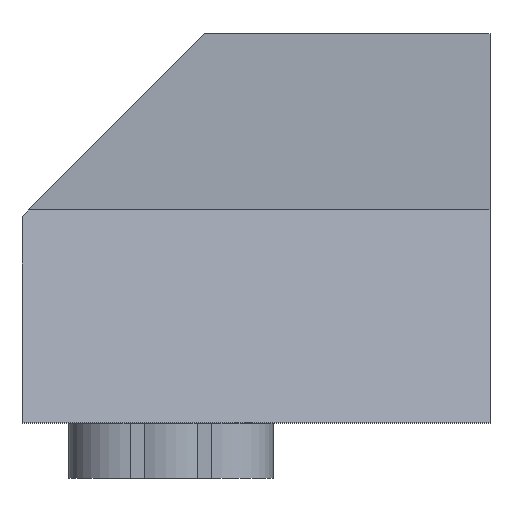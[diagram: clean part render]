
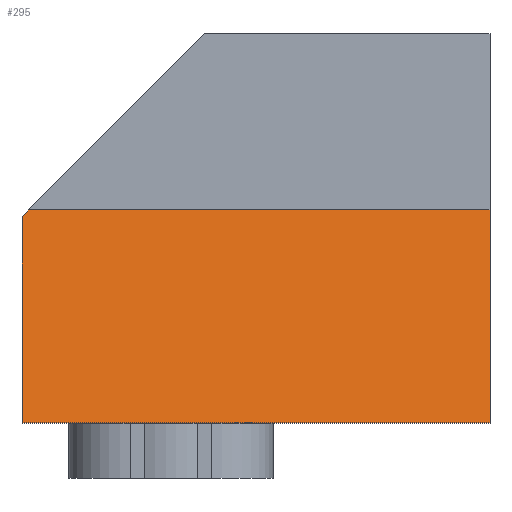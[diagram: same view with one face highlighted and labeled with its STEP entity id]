
A CAD part, left-side view. The second image highlights one B-rep face of the part: STEP entity #295.
In plain terms, the highlighted planar face has unit normal (-0.981, 0, 0.196).
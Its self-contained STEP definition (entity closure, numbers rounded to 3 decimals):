
#40 = VERTEX_POINT('',#41);
#41 = CARTESIAN_POINT('',(-1.5,-7.5,5.005));
#80 = EDGE_CURVE('',#81,#40,#83,.T.);
#81 = VERTEX_POINT('',#82);
#82 = CARTESIAN_POINT('',(-2.5,-7.5,0.005));
#83 = LINE('',#84,#85);
#84 = CARTESIAN_POINT('',(-2.5,-7.5,0.005));
#85 = VECTOR('',#86,1.);
#86 = DIRECTION('',(0.196,0.,0.981));
#276 = EDGE_CURVE('',#277,#81,#279,.T.);
#277 = VERTEX_POINT('',#278);
#278 = CARTESIAN_POINT('',(-2.5,3.5,0.005));
#279 = LINE('',#280,#281);
#280 = CARTESIAN_POINT('',(-2.5,3.5,0.005));
#281 = VECTOR('',#282,1.);
#282 = DIRECTION('',(0.,-1.,0.));
#295 = ADVANCED_FACE('',(#296),#322,.T.);
#296 = FACE_BOUND('',#297,.T.);
#297 = EDGE_LOOP('',(#298,#306,#314,#320,#321));
#298 = ORIENTED_EDGE('',*,*,#299,.F.);
#299 = EDGE_CURVE('',#300,#40,#302,.T.);
#300 = VERTEX_POINT('',#301);
#301 = CARTESIAN_POINT('',(-1.5,3.338,5.005));
#302 = LINE('',#303,#304);
#303 = CARTESIAN_POINT('',(-1.5,3.5,5.005));
#304 = VECTOR('',#305,1.);
#305 = DIRECTION('',(0.,-1.,0.));
#306 = ORIENTED_EDGE('',*,*,#307,.T.);
#307 = EDGE_CURVE('',#300,#308,#310,.T.);
#308 = VERTEX_POINT('',#309);
#309 = CARTESIAN_POINT('',(-1.532,3.5,4.843));
#310 = LINE('',#311,#312);
#311 = CARTESIAN_POINT('',(-1.455,3.114,5.229
    ));
#312 = VECTOR('',#313,1.);
#313 = DIRECTION('',(-0.14,0.7,-0.7));
#314 = ORIENTED_EDGE('',*,*,#315,.T.);
#315 = EDGE_CURVE('',#308,#277,#316,.T.);
#316 = LINE('',#317,#318);
#317 = CARTESIAN_POINT('',(-1.5,3.5,5.005));
#318 = VECTOR('',#319,1.);
#319 = DIRECTION('',(-0.196,0.,-0.981));
#320 = ORIENTED_EDGE('',*,*,#276,.T.);
#321 = ORIENTED_EDGE('',*,*,#80,.T.);
#322 = PLANE('',#323);
#323 = AXIS2_PLACEMENT_3D('',#324,#325,#326);
#324 = CARTESIAN_POINT('',(-2.,-2.,2.505));
#325 = DIRECTION('',(-0.981,0.,0.196)
  );
#326 = DIRECTION('',(-0.196,0.,-0.981
    ));
